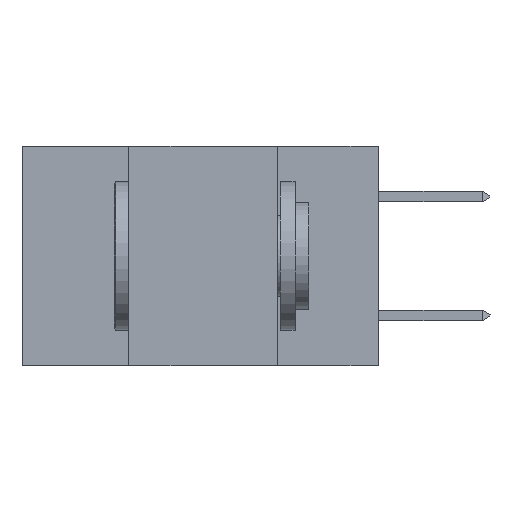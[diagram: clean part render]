
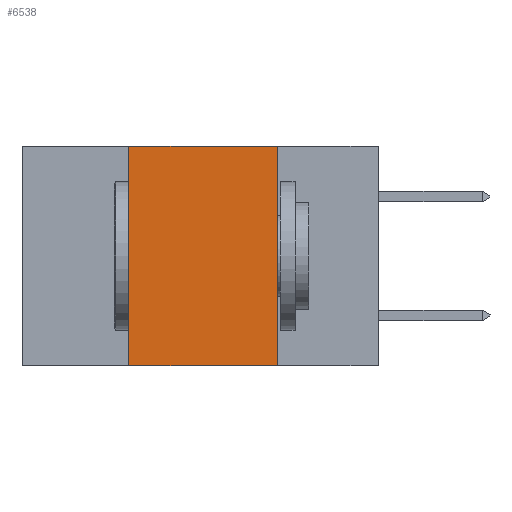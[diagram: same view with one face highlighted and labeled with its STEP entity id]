
A CAD part, left-side view. The second image highlights one B-rep face of the part: STEP entity #6538.
In plain terms, the highlighted planar face has unit normal (-1, 0, 0).
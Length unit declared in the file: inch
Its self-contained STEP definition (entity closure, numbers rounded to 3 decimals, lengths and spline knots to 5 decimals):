
#2137 = DIRECTION ( 'NONE',  ( 0., 0., -1. ) ) ;
#2845 = CARTESIAN_POINT ( 'NONE',  ( 0., 0.42, -0.37 ) ) ;
#3861 = EDGE_CURVE ( 'NONE', #18968, #5747, #6106, .T. ) ;
#4013 = CARTESIAN_POINT ( 'NONE',  ( 0., 0.42, 0. ) ) ;
#5216 = EDGE_CURVE ( 'NONE', #6115, #5747, #10850, .T. ) ;
#5747 = VERTEX_POINT ( 'NONE', #14833 ) ;
#5885 = ORIENTED_EDGE ( 'NONE', *, *, #18601, .F. ) ;
#6106 = LINE ( 'NONE', #14325, #24325 ) ;
#6115 = VERTEX_POINT ( 'NONE', #31611 ) ;
#6365 = ORIENTED_EDGE ( 'NONE', *, *, #7590, .F. ) ;
#6538 = ADVANCED_FACE ( 'NONE', ( #25365 ), #15242, .F. ) ;
#7096 = VECTOR ( 'NONE', #11695, 39.37008 ) ;
#7590 = EDGE_CURVE ( 'NONE', #28430, #6115, #18448, .T. ) ;
#10850 = LINE ( 'NONE', #12454, #13309 ) ;
#11362 = ORIENTED_EDGE ( 'NONE', *, *, #3861, .T. ) ;
#11457 = DIRECTION ( 'NONE',  ( 0., -1., 0. ) ) ;
#11695 = DIRECTION ( 'NONE',  ( 0., -1., 0. ) ) ;
#11909 = LINE ( 'NONE', #4013, #17196 ) ;
#12454 = CARTESIAN_POINT ( 'NONE',  ( 0., 0.17, 0. ) ) ;
#13309 = VECTOR ( 'NONE', #2137, 39.37008 ) ;
#14325 = CARTESIAN_POINT ( 'NONE',  ( 0., 0.6, -0.37 ) ) ;
#14833 = CARTESIAN_POINT ( 'NONE',  ( 0., 0.17, -0.37 ) ) ;
#14904 = CARTESIAN_POINT ( 'NONE',  ( 0., 0.6, 0. ) ) ;
#15242 = PLANE ( 'NONE',  #23524 ) ;
#17196 = VECTOR ( 'NONE', #19876, 39.37008 ) ;
#18448 = LINE ( 'NONE', #26760, #7096 ) ;
#18601 = EDGE_CURVE ( 'NONE', #18968, #28430, #11909, .T. ) ;
#18968 = VERTEX_POINT ( 'NONE', #2845 ) ;
#19876 = DIRECTION ( 'NONE',  ( 0., 0., 1. ) ) ;
#20305 = DIRECTION ( 'NONE',  ( 1., 0., 0. ) ) ;
#20534 = CARTESIAN_POINT ( 'NONE',  ( 0., 0.42, 0. ) ) ;
#23524 = AXIS2_PLACEMENT_3D ( 'NONE', #14904, #20305, #33291 ) ;
#24325 = VECTOR ( 'NONE', #11457, 39.37008 ) ;
#25365 = FACE_OUTER_BOUND ( 'NONE', #30092, .T. ) ;
#26760 = CARTESIAN_POINT ( 'NONE',  ( 0., 0.6, 0. ) ) ;
#27911 = ORIENTED_EDGE ( 'NONE', *, *, #5216, .F. ) ;
#28430 = VERTEX_POINT ( 'NONE', #20534 ) ;
#30092 = EDGE_LOOP ( 'NONE', ( #27911, #6365, #5885, #11362 ) ) ;
#31611 = CARTESIAN_POINT ( 'NONE',  ( 0., 0.17, 0. ) ) ;
#33291 = DIRECTION ( 'NONE',  ( 0., 0., -1. ) ) ;
